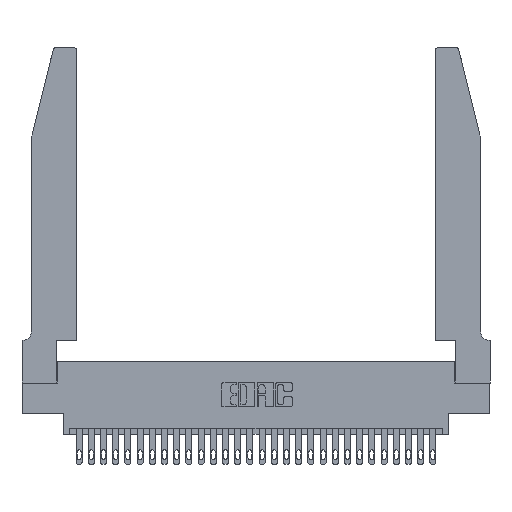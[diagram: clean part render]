
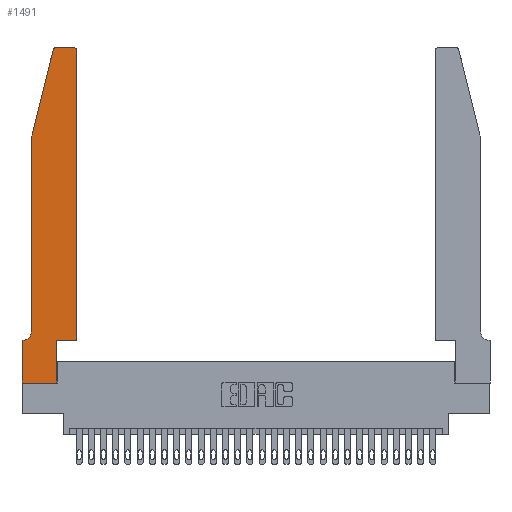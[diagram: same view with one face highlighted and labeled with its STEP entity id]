
A CAD part, top view. The second image highlights one B-rep face of the part: STEP entity #1491.
In plain terms, the highlighted planar face has unit normal (0, 0, 1).
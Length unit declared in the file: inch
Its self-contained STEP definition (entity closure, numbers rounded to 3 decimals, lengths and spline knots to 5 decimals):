
#246 = VECTOR ( 'NONE', #5131, 39.37008 ) ;
#925 = CARTESIAN_POINT ( 'NONE',  ( 0.2605, 2.75, 0.37 ) ) ;
#996 = VERTEX_POINT ( 'NONE', #27898 ) ;
#1179 = EDGE_CURVE ( 'NONE', #24379, #17388, #29909, .T. ) ;
#1491 = ADVANCED_FACE ( 'NONE', ( #28026 ), #6011, .T. ) ;
#1614 = ORIENTED_EDGE ( 'NONE', *, *, #19993, .T. ) ;
#1701 = DIRECTION ( 'NONE',  ( 1., 0., 0. ) ) ;
#2136 = ORIENTED_EDGE ( 'NONE', *, *, #11637, .T. ) ;
#2778 = CARTESIAN_POINT ( 'NONE',  ( 0.2865, 0., 0.37 ) ) ;
#2845 = VECTOR ( 'NONE', #11282, 39.37008 ) ;
#2930 = CARTESIAN_POINT ( 'NONE',  ( 0., 0., 0.37 ) ) ;
#3136 = CIRCLE ( 'NONE', #23886, 0.03 ) ;
#3651 = DIRECTION ( 'NONE',  ( -1., 0., 0. ) ) ;
#3694 = CARTESIAN_POINT ( 'NONE',  ( 0.4505, 0.35, 0.37 ) ) ;
#3766 = VECTOR ( 'NONE', #14303, 39.37008 ) ;
#4625 = DIRECTION ( 'NONE',  ( -1., 0., 0. ) ) ;
#5131 = DIRECTION ( 'NONE',  ( 1., 0., 0. ) ) ;
#5831 = CARTESIAN_POINT ( 'NONE',  ( 0.0755, 0.42, 0.37 ) ) ;
#5898 = EDGE_CURVE ( 'NONE', #17388, #10743, #12880, .T. ) ;
#5997 = VERTEX_POINT ( 'NONE', #5831 ) ;
#6011 = PLANE ( 'NONE',  #17441 ) ;
#6773 = VECTOR ( 'NONE', #12399, 39.37008 ) ;
#7597 = VECTOR ( 'NONE', #3651, 39.37008 ) ;
#8306 = LINE ( 'NONE', #9019, #7597 ) ;
#8307 = CARTESIAN_POINT ( 'NONE',  ( 0., 0.35, 0.37 ) ) ;
#8657 = VERTEX_POINT ( 'NONE', #24779 ) ;
#9019 = CARTESIAN_POINT ( 'NONE',  ( 0.0755, 0.35, 0.37 ) ) ;
#9078 = DIRECTION ( 'NONE',  ( 0., 0., -1. ) ) ;
#9269 = EDGE_CURVE ( 'NONE', #996, #14867, #8306, .T. ) ;
#9555 = CARTESIAN_POINT ( 'NONE',  ( 0.0755, 2., 0.37 ) ) ;
#10686 = CARTESIAN_POINT ( 'NONE',  ( 0.4505, 0.35, 0.37 ) ) ;
#10743 = VERTEX_POINT ( 'NONE', #12866 ) ;
#10942 = ORIENTED_EDGE ( 'NONE', *, *, #21886, .T. ) ;
#11282 = DIRECTION ( 'NONE',  ( 0., 1., 0. ) ) ;
#11637 = EDGE_CURVE ( 'NONE', #19811, #24379, #24078, .T. ) ;
#11990 = CARTESIAN_POINT ( 'NONE',  ( 0.4205, 2.72, 0.37 ) ) ;
#12086 = DIRECTION ( 'NONE',  ( 1., 0., 0. ) ) ;
#12386 = ORIENTED_EDGE ( 'NONE', *, *, #22183, .T. ) ;
#12399 = DIRECTION ( 'NONE',  ( -1., 0., 0. ) ) ;
#12486 = VERTEX_POINT ( 'NONE', #25628 ) ;
#12508 = CARTESIAN_POINT ( 'NONE',  ( 0., 0., 0.37 ) ) ;
#12866 = CARTESIAN_POINT ( 'NONE',  ( 0.284, 2.75, 0.37 ) ) ;
#12880 = LINE ( 'NONE', #925, #6773 ) ;
#13200 = EDGE_CURVE ( 'NONE', #5997, #996, #29454, .T. ) ;
#13320 = ORIENTED_EDGE ( 'NONE', *, *, #1179, .T. ) ;
#13654 = LINE ( 'NONE', #13869, #2845 ) ;
#13869 = CARTESIAN_POINT ( 'NONE',  ( 0.2865, 0.35, 0.37 ) ) ;
#14048 = EDGE_CURVE ( 'NONE', #14867, #27740, #26708, .T. ) ;
#14303 = DIRECTION ( 'NONE',  ( 0., -1., 0. ) ) ;
#14363 = ORIENTED_EDGE ( 'NONE', *, *, #20788, .T. ) ;
#14867 = VERTEX_POINT ( 'NONE', #29221 ) ;
#15300 = CARTESIAN_POINT ( 'NONE',  ( 0.4205, 2.75, 0.37 ) ) ;
#15423 = ORIENTED_EDGE ( 'NONE', *, *, #23299, .T. ) ;
#15893 = AXIS2_PLACEMENT_3D ( 'NONE', #11990, #16729, #12086 ) ;
#15909 = ORIENTED_EDGE ( 'NONE', *, *, #5898, .T. ) ;
#16146 = ORIENTED_EDGE ( 'NONE', *, *, #9269, .T. ) ;
#16729 = DIRECTION ( 'NONE',  ( 0., 0., 1. ) ) ;
#17388 = VERTEX_POINT ( 'NONE', #15300 ) ;
#17441 = AXIS2_PLACEMENT_3D ( 'NONE', #8307, #26866, #1701 ) ;
#18247 = VERTEX_POINT ( 'NONE', #2778 ) ;
#19479 = ORIENTED_EDGE ( 'NONE', *, *, #14048, .T. ) ;
#19748 = CARTESIAN_POINT ( 'NONE',  ( 0.4505, 2.72, 0.37 ) ) ;
#19811 = VERTEX_POINT ( 'NONE', #3694 ) ;
#19993 = EDGE_CURVE ( 'NONE', #8657, #22719, #26030, .T. ) ;
#20116 = EDGE_CURVE ( 'NONE', #12486, #19811, #22005, .T. ) ;
#20132 = DIRECTION ( 'NONE',  ( -0.239, -0.971, 0. ) ) ;
#20314 = DIRECTION ( 'NONE',  ( 0., 1., 0. ) ) ;
#20788 = EDGE_CURVE ( 'NONE', #18247, #12486, #13654, .T. ) ;
#21292 = VECTOR ( 'NONE', #24544, 39.37008 ) ;
#21886 = EDGE_CURVE ( 'NONE', #10743, #8657, #3136, .T. ) ;
#21953 = ORIENTED_EDGE ( 'NONE', *, *, #13200, .T. ) ;
#22005 = LINE ( 'NONE', #10686, #21292 ) ;
#22183 = EDGE_CURVE ( 'NONE', #27740, #18247, #26640, .T. ) ;
#22188 = LINE ( 'NONE', #9555, #3766 ) ;
#22710 = VECTOR ( 'NONE', #28832, 39.37008 ) ;
#22719 = VERTEX_POINT ( 'NONE', #23475 ) ;
#22730 = DIRECTION ( 'NONE',  ( 0., 0., 1. ) ) ;
#23299 = EDGE_CURVE ( 'NONE', #22719, #5997, #22188, .T. ) ;
#23346 = AXIS2_PLACEMENT_3D ( 'NONE', #28548, #9078, #4625 ) ;
#23475 = CARTESIAN_POINT ( 'NONE',  ( 0.0755, 2., 0.37 ) ) ;
#23881 = EDGE_LOOP ( 'NONE', ( #15909, #10942, #1614, #15423, #21953, #16146, #19479, #12386, #14363, #24819, #2136, #13320 ) ) ;
#23886 = AXIS2_PLACEMENT_3D ( 'NONE', #24875, #22730, #25087 ) ;
#24078 = LINE ( 'NONE', #29915, #27375 ) ;
#24379 = VERTEX_POINT ( 'NONE', #19748 ) ;
#24544 = DIRECTION ( 'NONE',  ( 1., 0., 0. ) ) ;
#24779 = CARTESIAN_POINT ( 'NONE',  ( 0.25487, 2.72718, 0.37 ) ) ;
#24819 = ORIENTED_EDGE ( 'NONE', *, *, #20116, .T. ) ;
#24829 = CARTESIAN_POINT ( 'NONE',  ( 0.0755, 2., 0.37 ) ) ;
#24875 = CARTESIAN_POINT ( 'NONE',  ( 0.284, 2.72, 0.37 ) ) ;
#25087 = DIRECTION ( 'NONE',  ( 1., 0., 0. ) ) ;
#25398 = CARTESIAN_POINT ( 'NONE',  ( 0., 0., 0.37 ) ) ;
#25628 = CARTESIAN_POINT ( 'NONE',  ( 0.2865, 0.35, 0.37 ) ) ;
#26030 = LINE ( 'NONE', #24829, #28215 ) ;
#26640 = LINE ( 'NONE', #2930, #246 ) ;
#26708 = LINE ( 'NONE', #12508, #22710 ) ;
#26866 = DIRECTION ( 'NONE',  ( 0., 0., 1. ) ) ;
#27375 = VECTOR ( 'NONE', #20314, 39.37008 ) ;
#27740 = VERTEX_POINT ( 'NONE', #25398 ) ;
#27898 = CARTESIAN_POINT ( 'NONE',  ( 0.0055, 0.35, 0.37 ) ) ;
#28026 = FACE_OUTER_BOUND ( 'NONE', #23881, .T. ) ;
#28215 = VECTOR ( 'NONE', #20132, 39.37008 ) ;
#28548 = CARTESIAN_POINT ( 'NONE',  ( 0.0055, 0.42, 0.37 ) ) ;
#28832 = DIRECTION ( 'NONE',  ( 0., -1., 0. ) ) ;
#29221 = CARTESIAN_POINT ( 'NONE',  ( 0., 0.35, 0.37 ) ) ;
#29454 = CIRCLE ( 'NONE', #23346, 0.07 ) ;
#29909 = CIRCLE ( 'NONE', #15893, 0.03 ) ;
#29915 = CARTESIAN_POINT ( 'NONE',  ( 0.4505, 0.35, 0.37 ) ) ;
